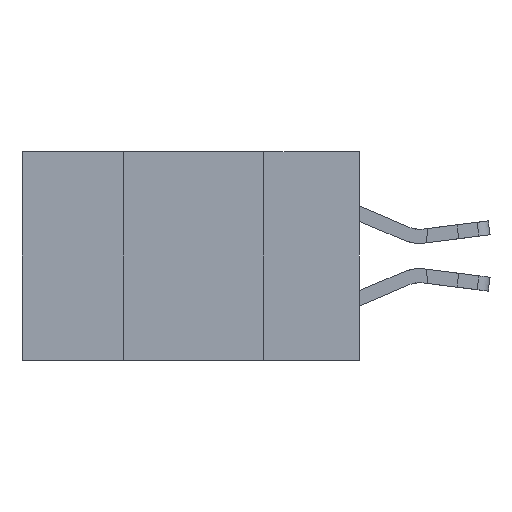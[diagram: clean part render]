
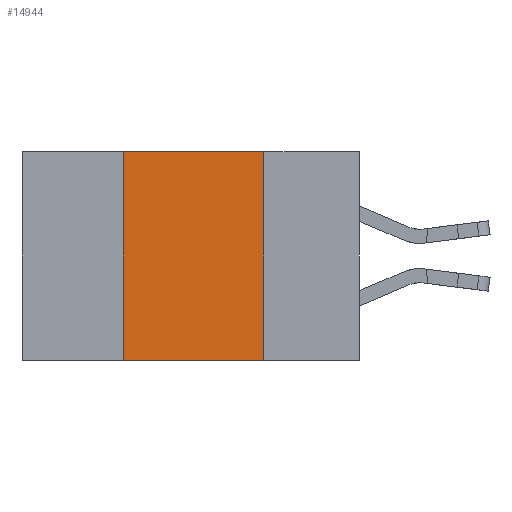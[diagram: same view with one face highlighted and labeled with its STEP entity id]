
A CAD part, left-side view. The second image highlights one B-rep face of the part: STEP entity #14944.
In plain terms, the highlighted planar face has unit normal (-1, 0, 0).
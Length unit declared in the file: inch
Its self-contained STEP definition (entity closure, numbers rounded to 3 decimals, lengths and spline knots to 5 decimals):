
#207 = CARTESIAN_POINT ( 'NONE',  ( 0., 0.42, 0. ) ) ;
#836 = ORIENTED_EDGE ( 'NONE', *, *, #13838, .T. ) ;
#1094 = VECTOR ( 'NONE', #10273, 39.37008 ) ;
#1190 = CARTESIAN_POINT ( 'NONE',  ( 0., 0.17, 0. ) ) ;
#1839 = EDGE_CURVE ( 'NONE', #12145, #15596, #9786, .T. ) ;
#1875 = ORIENTED_EDGE ( 'NONE', *, *, #15108, .F. ) ;
#2339 = EDGE_CURVE ( 'NONE', #10800, #8851, #6777, .T. ) ;
#2861 = VECTOR ( 'NONE', #11124, 39.37008 ) ;
#3188 = LINE ( 'NONE', #7300, #1094 ) ;
#4012 = AXIS2_PLACEMENT_3D ( 'NONE', #8655, #18954, #10130 ) ;
#4117 = CARTESIAN_POINT ( 'NONE',  ( 0., 0.6, -0.37 ) ) ;
#4414 = CARTESIAN_POINT ( 'NONE',  ( 0., 0.42, -0.37 ) ) ;
#4826 = LINE ( 'NONE', #4117, #6896 ) ;
#5071 = FACE_OUTER_BOUND ( 'NONE', #5099, .T. ) ;
#5099 = EDGE_LOOP ( 'NONE', ( #14368, #1875, #5592, #836 ) ) ;
#5592 = ORIENTED_EDGE ( 'NONE', *, *, #1839, .F. ) ;
#6516 = CARTESIAN_POINT ( 'NONE',  ( 0., 0.42, 0. ) ) ;
#6777 = LINE ( 'NONE', #6906, #2861 ) ;
#6896 = VECTOR ( 'NONE', #18614, 39.37008 ) ;
#6906 = CARTESIAN_POINT ( 'NONE',  ( 0., 0.17, 0. ) ) ;
#7300 = CARTESIAN_POINT ( 'NONE',  ( 0., 0.6, 0. ) ) ;
#8655 = CARTESIAN_POINT ( 'NONE',  ( 0., 0.6, 0. ) ) ;
#8851 = VERTEX_POINT ( 'NONE', #8965 ) ;
#8965 = CARTESIAN_POINT ( 'NONE',  ( 0., 0.17, -0.37 ) ) ;
#9786 = LINE ( 'NONE', #207, #13268 ) ;
#10130 = DIRECTION ( 'NONE',  ( 0., 0., -1. ) ) ;
#10273 = DIRECTION ( 'NONE',  ( 0., -1., 0. ) ) ;
#10800 = VERTEX_POINT ( 'NONE', #1190 ) ;
#11124 = DIRECTION ( 'NONE',  ( 0., 0., -1. ) ) ;
#12145 = VERTEX_POINT ( 'NONE', #4414 ) ;
#13268 = VECTOR ( 'NONE', #13541, 39.37008 ) ;
#13541 = DIRECTION ( 'NONE',  ( 0., 0., 1. ) ) ;
#13838 = EDGE_CURVE ( 'NONE', #12145, #8851, #4826, .T. ) ;
#14322 = PLANE ( 'NONE',  #4012 ) ;
#14368 = ORIENTED_EDGE ( 'NONE', *, *, #2339, .F. ) ;
#14944 = ADVANCED_FACE ( 'NONE', ( #5071 ), #14322, .F. ) ;
#15108 = EDGE_CURVE ( 'NONE', #15596, #10800, #3188, .T. ) ;
#15596 = VERTEX_POINT ( 'NONE', #6516 ) ;
#18614 = DIRECTION ( 'NONE',  ( 0., -1., 0. ) ) ;
#18954 = DIRECTION ( 'NONE',  ( 1., 0., 0. ) ) ;
